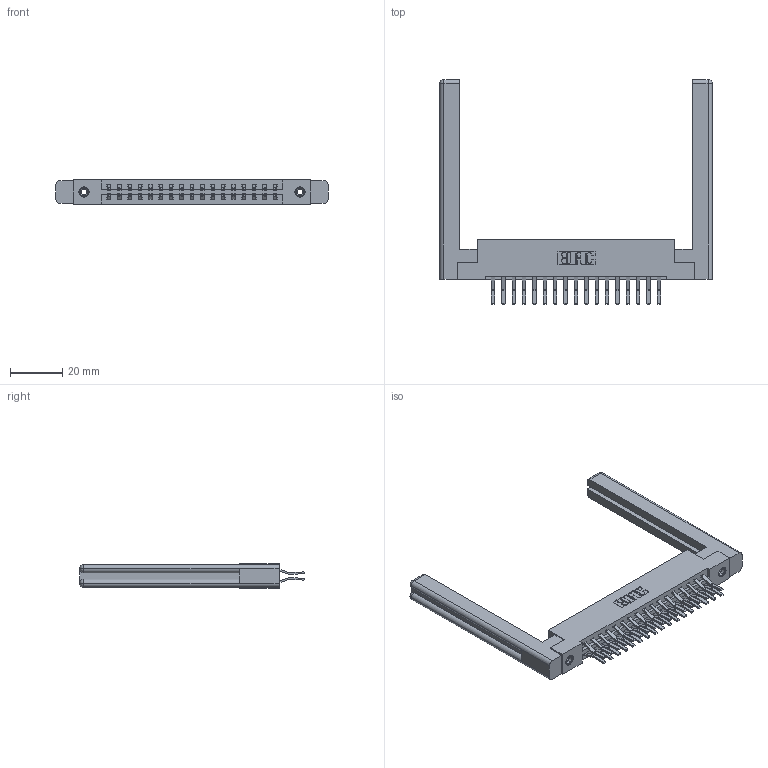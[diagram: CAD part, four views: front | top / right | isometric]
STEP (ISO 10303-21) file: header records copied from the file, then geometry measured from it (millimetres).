
FILE_DESCRIPTION (( 'STEP AP203' ), '1' );
FILE_NAME ('387-034-560-258.STEP', '2019-10-17T18:30:39', ( '' ), ( '' ), 'SwSTEP 2.0', 'SolidWorks 2016', '' );
FILE_SCHEMA (( 'CONFIG_CONTROL_DESIGN' ));
Length unit declared in the file: inch
Products named in the file (5): 307-220-058; 337 Part_Flush Mounting Lugs - 0.156 Dia-TI; 345-292-001_560 Tail; 387-034-560-258; 345-250-001_345-250-001-102
Assembly tree (39 placements, depth 2):
  387-034-560-258
    337 Part_Flush Mounting Lugs - 0.156 Dia-TI
    345-292-001_560 Tail  x34
    345-250-001_345-250-001-102  x2
    307-220-058  x2
Bounding box: 103.99 x 85.87 x 9.4 mm (x, y, z)
Volume: 17991.5 mm3; surface area: 17713.9 mm2
Topology: 39 solids, 39 shells, 2160 faces, 6343 edges, 4170 vertices
Faces by surface type: plane 1446, cylinder 690, cone 12, torus 12
Entity records: 19136 total; most frequent: CARTESIAN_POINT 3253, ORIENTED_EDGE 3128, DIRECTION 2832, EDGE_CURVE 1564, LINE 1384, VECTOR 1384, VERTEX_POINT 1034, AXIS2_PLACEMENT_3D 724
